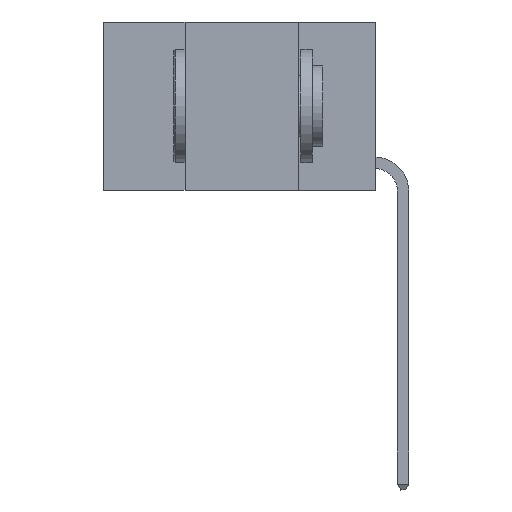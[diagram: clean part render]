
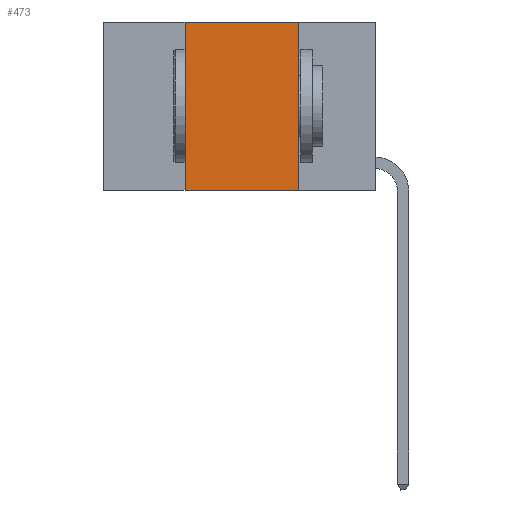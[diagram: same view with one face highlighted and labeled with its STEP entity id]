
A CAD part, left-side view. The second image highlights one B-rep face of the part: STEP entity #473.
In plain terms, the highlighted planar face has unit normal (-1, 0, 0).
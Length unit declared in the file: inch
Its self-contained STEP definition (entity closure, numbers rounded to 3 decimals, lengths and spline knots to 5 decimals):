
#222 = CARTESIAN_POINT ( 'NONE',  ( 0., 0.17, -0.37 ) ) ;
#460 = EDGE_CURVE ( 'NONE', #9014, #15112, #8915, .T. ) ;
#473 = ADVANCED_FACE ( 'NONE', ( #16818 ), #2751, .F. ) ;
#2093 = CARTESIAN_POINT ( 'NONE',  ( 0., 0.42, 0. ) ) ;
#2176 = DIRECTION ( 'NONE',  ( 0., 0., 1. ) ) ;
#2419 = CARTESIAN_POINT ( 'NONE',  ( 0., 0.6, -0.37 ) ) ;
#2580 = CARTESIAN_POINT ( 'NONE',  ( 0., 0.6, 0. ) ) ;
#2751 = PLANE ( 'NONE',  #15644 ) ;
#3489 = VERTEX_POINT ( 'NONE', #10719 ) ;
#3567 = EDGE_CURVE ( 'NONE', #15112, #3489, #8672, .T. ) ;
#4449 = ORIENTED_EDGE ( 'NONE', *, *, #460, .F. ) ;
#4859 = DIRECTION ( 'NONE',  ( 0., -1., 0. ) ) ;
#5296 = VERTEX_POINT ( 'NONE', #222 ) ;
#5711 = CARTESIAN_POINT ( 'NONE',  ( 0., 0.42, 0. ) ) ;
#5885 = ORIENTED_EDGE ( 'NONE', *, *, #15334, .T. ) ;
#5969 = VECTOR ( 'NONE', #2176, 39.37008 ) ;
#6233 = LINE ( 'NONE', #2419, #15011 ) ;
#6269 = ORIENTED_EDGE ( 'NONE', *, *, #6379, .F. ) ;
#6379 = EDGE_CURVE ( 'NONE', #3489, #5296, #14983, .T. ) ;
#7193 = CARTESIAN_POINT ( 'NONE',  ( 0., 0.17, 0. ) ) ;
#7290 = CARTESIAN_POINT ( 'NONE',  ( 0., 0.6, 0. ) ) ;
#7530 = VECTOR ( 'NONE', #4859, 39.37008 ) ;
#8670 = DIRECTION ( 'NONE',  ( 0., 0., -1. ) ) ;
#8672 = LINE ( 'NONE', #7290, #7530 ) ;
#8915 = LINE ( 'NONE', #2093, #5969 ) ;
#9014 = VERTEX_POINT ( 'NONE', #11614 ) ;
#10719 = CARTESIAN_POINT ( 'NONE',  ( 0., 0.17, 0. ) ) ;
#11501 = DIRECTION ( 'NONE',  ( 0., -1., 0. ) ) ;
#11614 = CARTESIAN_POINT ( 'NONE',  ( 0., 0.42, -0.37 ) ) ;
#11746 = DIRECTION ( 'NONE',  ( 0., 0., -1. ) ) ;
#12229 = ORIENTED_EDGE ( 'NONE', *, *, #3567, .F. ) ;
#13320 = DIRECTION ( 'NONE',  ( 1., 0., 0. ) ) ;
#14541 = EDGE_LOOP ( 'NONE', ( #6269, #12229, #4449, #5885 ) ) ;
#14983 = LINE ( 'NONE', #7193, #15466 ) ;
#15011 = VECTOR ( 'NONE', #11501, 39.37008 ) ;
#15112 = VERTEX_POINT ( 'NONE', #5711 ) ;
#15334 = EDGE_CURVE ( 'NONE', #9014, #5296, #6233, .T. ) ;
#15466 = VECTOR ( 'NONE', #8670, 39.37008 ) ;
#15644 = AXIS2_PLACEMENT_3D ( 'NONE', #2580, #13320, #11746 ) ;
#16818 = FACE_OUTER_BOUND ( 'NONE', #14541, .T. ) ;
